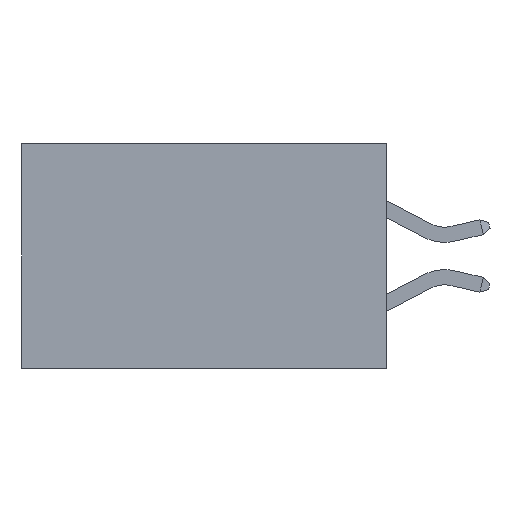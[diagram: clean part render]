
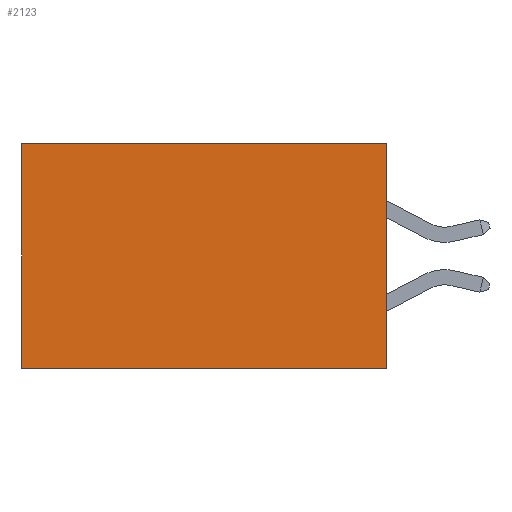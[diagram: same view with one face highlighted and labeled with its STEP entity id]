
A CAD part, left-side view. The second image highlights one B-rep face of the part: STEP entity #2123.
In plain terms, the highlighted planar face has unit normal (-1, 0, 0).
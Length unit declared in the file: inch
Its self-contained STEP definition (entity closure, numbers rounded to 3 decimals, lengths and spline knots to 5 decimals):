
#440 = CARTESIAN_POINT ( 'NONE',  ( 0.298, 0.6, 0. ) ) ;
#641 = EDGE_CURVE ( 'NONE', #17822, #4004, #11398, .T. ) ;
#1924 = ORIENTED_EDGE ( 'NONE', *, *, #9863, .T. ) ;
#2123 = ADVANCED_FACE ( 'NONE', ( #17468 ), #10658, .F. ) ;
#2432 = LINE ( 'NONE', #5787, #5785 ) ;
#2925 = VECTOR ( 'NONE', #5210, 39.37008 ) ;
#2930 = CARTESIAN_POINT ( 'NONE',  ( 0.298, 0., 0. ) ) ;
#3197 = DIRECTION ( 'NONE',  ( 0., 0., -1. ) ) ;
#3594 = CARTESIAN_POINT ( 'NONE',  ( 0.298, 0., 0. ) ) ;
#4004 = VERTEX_POINT ( 'NONE', #18044 ) ;
#5210 = DIRECTION ( 'NONE',  ( 0., 0., -1. ) ) ;
#5785 = VECTOR ( 'NONE', #17034, 39.37008 ) ;
#5787 = CARTESIAN_POINT ( 'NONE',  ( 0.298, 0., -0.37 ) ) ;
#6300 = LINE ( 'NONE', #9435, #2925 ) ;
#7933 = VECTOR ( 'NONE', #12088, 39.37008 ) ;
#8364 = LINE ( 'NONE', #3594, #7933 ) ;
#9435 = CARTESIAN_POINT ( 'NONE',  ( 0.298, 0.6, 0. ) ) ;
#9863 = EDGE_CURVE ( 'NONE', #17822, #16325, #8364, .T. ) ;
#10305 = CARTESIAN_POINT ( 'NONE',  ( 0.298, 0., 0. ) ) ;
#10658 = PLANE ( 'NONE',  #13405 ) ;
#11398 = LINE ( 'NONE', #2930, #15148 ) ;
#11725 = ORIENTED_EDGE ( 'NONE', *, *, #641, .F. ) ;
#11794 = CARTESIAN_POINT ( 'NONE',  ( 0.298, 0.6, -0.37 ) ) ;
#12088 = DIRECTION ( 'NONE',  ( 0., 1., 0. ) ) ;
#13405 = AXIS2_PLACEMENT_3D ( 'NONE', #10305, #13560, #3197 ) ;
#13560 = DIRECTION ( 'NONE',  ( 1., 0., 0. ) ) ;
#13843 = EDGE_CURVE ( 'NONE', #4004, #17418, #2432, .T. ) ;
#14497 = ORIENTED_EDGE ( 'NONE', *, *, #15310, .T. ) ;
#15148 = VECTOR ( 'NONE', #16336, 39.37008 ) ;
#15271 = EDGE_LOOP ( 'NONE', ( #14497, #16558, #11725, #1924 ) ) ;
#15310 = EDGE_CURVE ( 'NONE', #16325, #17418, #6300, .T. ) ;
#15417 = CARTESIAN_POINT ( 'NONE',  ( 0.298, 0., 0. ) ) ;
#16325 = VERTEX_POINT ( 'NONE', #440 ) ;
#16336 = DIRECTION ( 'NONE',  ( 0., 0., -1. ) ) ;
#16558 = ORIENTED_EDGE ( 'NONE', *, *, #13843, .F. ) ;
#17034 = DIRECTION ( 'NONE',  ( 0., 1., 0. ) ) ;
#17418 = VERTEX_POINT ( 'NONE', #11794 ) ;
#17468 = FACE_OUTER_BOUND ( 'NONE', #15271, .T. ) ;
#17822 = VERTEX_POINT ( 'NONE', #15417 ) ;
#18044 = CARTESIAN_POINT ( 'NONE',  ( 0.298, 0., -0.37 ) ) ;
